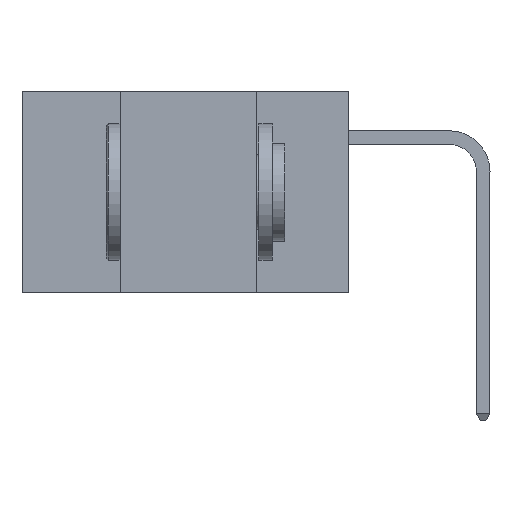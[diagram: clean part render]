
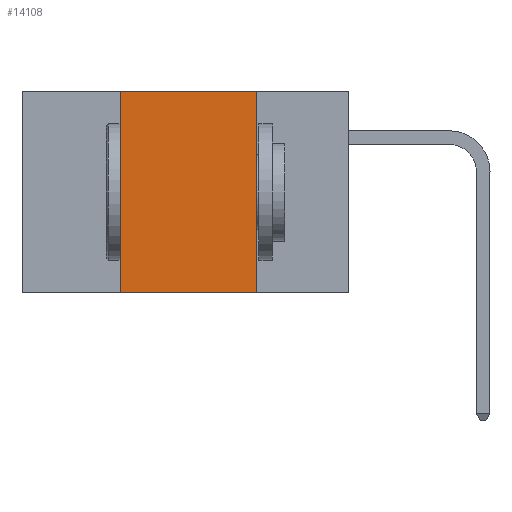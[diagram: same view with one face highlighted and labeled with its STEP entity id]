
A CAD part, left-side view. The second image highlights one B-rep face of the part: STEP entity #14108.
In plain terms, the highlighted planar face has unit normal (-1, 0, 0).
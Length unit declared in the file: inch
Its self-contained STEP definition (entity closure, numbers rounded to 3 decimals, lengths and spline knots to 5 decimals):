
#1107 = ORIENTED_EDGE ( 'NONE', *, *, #25018, .F. ) ;
#1149 = CARTESIAN_POINT ( 'NONE',  ( 0., 0.42, 0. ) ) ;
#1262 = ORIENTED_EDGE ( 'NONE', *, *, #26866, .F. ) ;
#1413 = LINE ( 'NONE', #18025, #24653 ) ;
#1512 = LINE ( 'NONE', #1149, #14606 ) ;
#2214 = AXIS2_PLACEMENT_3D ( 'NONE', #8241, #10662, #26905 ) ;
#2830 = EDGE_CURVE ( 'NONE', #11691, #17171, #1512, .T. ) ;
#3721 = PLANE ( 'NONE',  #2214 ) ;
#4061 = DIRECTION ( 'NONE',  ( 0., 0., -1. ) ) ;
#4256 = VECTOR ( 'NONE', #26839, 39.37008 ) ;
#4534 = FACE_OUTER_BOUND ( 'NONE', #14620, .T. ) ;
#5260 = EDGE_CURVE ( 'NONE', #11691, #7987, #17382, .T. ) ;
#7987 = VERTEX_POINT ( 'NONE', #15463 ) ;
#8241 = CARTESIAN_POINT ( 'NONE',  ( 0., 0.6, 0. ) ) ;
#8273 = CARTESIAN_POINT ( 'NONE',  ( 0., 0.6, -0.37 ) ) ;
#9868 = ORIENTED_EDGE ( 'NONE', *, *, #5260, .T. ) ;
#10662 = DIRECTION ( 'NONE',  ( 1., 0., 0. ) ) ;
#11121 = CARTESIAN_POINT ( 'NONE',  ( 0., 0.6, 0. ) ) ;
#11691 = VERTEX_POINT ( 'NONE', #14820 ) ;
#13328 = CARTESIAN_POINT ( 'NONE',  ( 0., 0.17, 0. ) ) ;
#14108 = ADVANCED_FACE ( 'NONE', ( #4534 ), #3721, .F. ) ;
#14606 = VECTOR ( 'NONE', #17450, 39.37008 ) ;
#14620 = EDGE_LOOP ( 'NONE', ( #1107, #1262, #15449, #9868 ) ) ;
#14820 = CARTESIAN_POINT ( 'NONE',  ( 0., 0.42, -0.37 ) ) ;
#15449 = ORIENTED_EDGE ( 'NONE', *, *, #2830, .F. ) ;
#15463 = CARTESIAN_POINT ( 'NONE',  ( 0., 0.17, -0.37 ) ) ;
#17171 = VERTEX_POINT ( 'NONE', #22626 ) ;
#17382 = LINE ( 'NONE', #8273, #4256 ) ;
#17450 = DIRECTION ( 'NONE',  ( 0., 0., 1. ) ) ;
#18025 = CARTESIAN_POINT ( 'NONE',  ( 0., 0.17, 0. ) ) ;
#19300 = VECTOR ( 'NONE', #25050, 39.37008 ) ;
#20855 = VERTEX_POINT ( 'NONE', #13328 ) ;
#22626 = CARTESIAN_POINT ( 'NONE',  ( 0., 0.42, 0. ) ) ;
#24653 = VECTOR ( 'NONE', #4061, 39.37008 ) ;
#25018 = EDGE_CURVE ( 'NONE', #20855, #7987, #1413, .T. ) ;
#25050 = DIRECTION ( 'NONE',  ( 0., -1., 0. ) ) ;
#25375 = LINE ( 'NONE', #11121, #19300 ) ;
#26839 = DIRECTION ( 'NONE',  ( 0., -1., 0. ) ) ;
#26866 = EDGE_CURVE ( 'NONE', #17171, #20855, #25375, .T. ) ;
#26905 = DIRECTION ( 'NONE',  ( 0., 0., -1. ) ) ;
